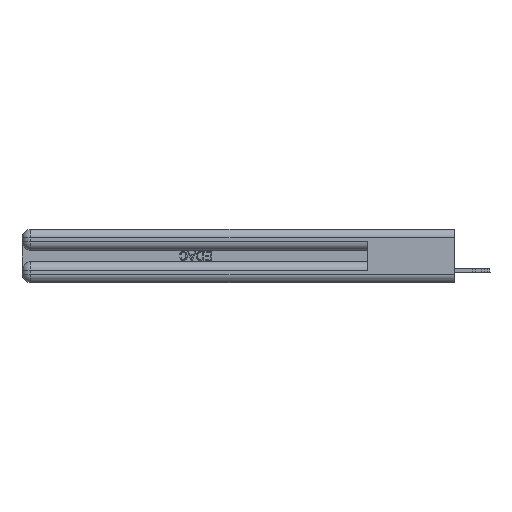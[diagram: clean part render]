
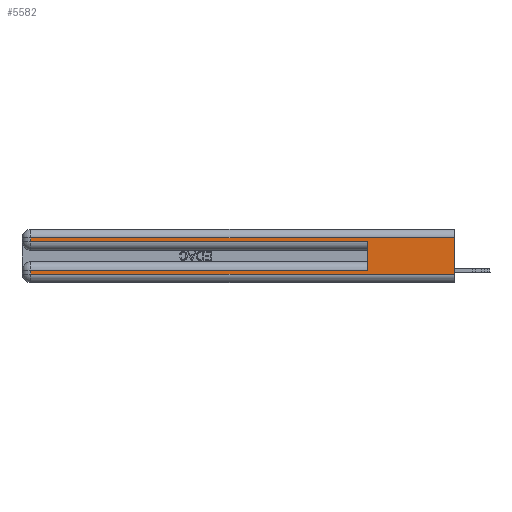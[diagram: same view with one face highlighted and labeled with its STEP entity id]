
A CAD part, left-side view. The second image highlights one B-rep face of the part: STEP entity #5582.
In plain terms, the highlighted planar face has unit normal (-1, 0, 0).
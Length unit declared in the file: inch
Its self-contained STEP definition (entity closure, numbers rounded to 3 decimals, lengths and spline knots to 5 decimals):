
#443 = VECTOR ( 'NONE', #26370, 39.37008 ) ;
#1154 = LINE ( 'NONE', #27697, #9034 ) ;
#2442 = DIRECTION ( 'NONE',  ( 1., 0., 0. ) ) ;
#3306 = VERTEX_POINT ( 'NONE', #29395 ) ;
#4145 = VECTOR ( 'NONE', #40556, 39.37008 ) ;
#4469 = ORIENTED_EDGE ( 'NONE', *, *, #9109, .T. ) ;
#4774 = EDGE_LOOP ( 'NONE', ( #36226, #4469, #39817, #7305, #7699, #21751, #13454, #14660 ) ) ;
#5394 = DIRECTION ( 'NONE',  ( 0., 0., 1. ) ) ;
#5557 = VERTEX_POINT ( 'NONE', #19519 ) ;
#5582 = ADVANCED_FACE ( 'NONE', ( #32559 ), #15690, .F. ) ;
#7305 = ORIENTED_EDGE ( 'NONE', *, *, #16954, .T. ) ;
#7699 = ORIENTED_EDGE ( 'NONE', *, *, #25965, .F. ) ;
#9034 = VECTOR ( 'NONE', #38230, 39.37008 ) ;
#9109 = EDGE_CURVE ( 'NONE', #16203, #12851, #16235, .T. ) ;
#11168 = VECTOR ( 'NONE', #5394, 39.37008 ) ;
#12367 = CARTESIAN_POINT ( 'NONE',  ( 0., 2.94, 0.06 ) ) ;
#12851 = VERTEX_POINT ( 'NONE', #13276 ) ;
#13276 = CARTESIAN_POINT ( 'NONE',  ( 0., 2.94, 0.31 ) ) ;
#13454 = ORIENTED_EDGE ( 'NONE', *, *, #15266, .T. ) ;
#14408 = VECTOR ( 'NONE', #34751, 39.37008 ) ;
#14660 = ORIENTED_EDGE ( 'NONE', *, *, #39453, .T. ) ;
#15266 = EDGE_CURVE ( 'NONE', #39460, #23710, #37892, .T. ) ;
#15690 = PLANE ( 'NONE',  #36865 ) ;
#16203 = VERTEX_POINT ( 'NONE', #29167 ) ;
#16235 = LINE ( 'NONE', #23032, #443 ) ;
#16908 = CARTESIAN_POINT ( 'NONE',  ( 0., 0.6, 0.285 ) ) ;
#16954 = EDGE_CURVE ( 'NONE', #17671, #34526, #23064, .T. ) ;
#17656 = CARTESIAN_POINT ( 'NONE',  ( 0., 0., 0.37 ) ) ;
#17671 = VERTEX_POINT ( 'NONE', #28675 ) ;
#17697 = DIRECTION ( 'NONE',  ( 0., 0., -1. ) ) ;
#19519 = CARTESIAN_POINT ( 'NONE',  ( 0., 0., 0.06 ) ) ;
#19958 = VECTOR ( 'NONE', #39083, 39.37008 ) ;
#20696 = LINE ( 'NONE', #17656, #14408 ) ;
#20820 = EDGE_CURVE ( 'NONE', #12851, #17671, #36679, .T. ) ;
#20942 = CARTESIAN_POINT ( 'NONE',  ( 0., 2.94, 0.37 ) ) ;
#21751 = ORIENTED_EDGE ( 'NONE', *, *, #33394, .T. ) ;
#22437 = CARTESIAN_POINT ( 'NONE',  ( 0., 0., 0.37 ) ) ;
#23032 = CARTESIAN_POINT ( 'NONE',  ( 0., 0., 0.31 ) ) ;
#23064 = LINE ( 'NONE', #39695, #4145 ) ;
#23710 = VERTEX_POINT ( 'NONE', #12367 ) ;
#25199 = EDGE_CURVE ( 'NONE', #16203, #5557, #20696, .T. ) ;
#25965 = EDGE_CURVE ( 'NONE', #3306, #34526, #36319, .T. ) ;
#26370 = DIRECTION ( 'NONE',  ( 0., 1., 0. ) ) ;
#27422 = LINE ( 'NONE', #32650, #33184 ) ;
#27697 = CARTESIAN_POINT ( 'NONE',  ( 0., 0., 0.085 ) ) ;
#28566 = CARTESIAN_POINT ( 'NONE',  ( 0., 0.6, 0.145 ) ) ;
#28675 = CARTESIAN_POINT ( 'NONE',  ( 0., 2.94, 0.285 ) ) ;
#29122 = DIRECTION ( 'NONE',  ( 0., -1., 0. ) ) ;
#29167 = CARTESIAN_POINT ( 'NONE',  ( 0., 0., 0.31 ) ) ;
#29395 = CARTESIAN_POINT ( 'NONE',  ( 0., 0.6, 0.085 ) ) ;
#31629 = VECTOR ( 'NONE', #17697, 39.37008 ) ;
#32559 = FACE_OUTER_BOUND ( 'NONE', #4774, .T. ) ;
#32650 = CARTESIAN_POINT ( 'NONE',  ( 0., 0., 0.06 ) ) ;
#33061 = CARTESIAN_POINT ( 'NONE',  ( 0., 2.94, 0.37 ) ) ;
#33184 = VECTOR ( 'NONE', #29122, 39.37008 ) ;
#33394 = EDGE_CURVE ( 'NONE', #3306, #39460, #1154, .T. ) ;
#34526 = VERTEX_POINT ( 'NONE', #16908 ) ;
#34751 = DIRECTION ( 'NONE',  ( 0., 0., -1. ) ) ;
#35587 = DIRECTION ( 'NONE',  ( 0., 0., -1. ) ) ;
#36226 = ORIENTED_EDGE ( 'NONE', *, *, #25199, .F. ) ;
#36319 = LINE ( 'NONE', #28566, #11168 ) ;
#36679 = LINE ( 'NONE', #33061, #19958 ) ;
#36865 = AXIS2_PLACEMENT_3D ( 'NONE', #22437, #2442, #35587 ) ;
#37892 = LINE ( 'NONE', #20942, #31629 ) ;
#38230 = DIRECTION ( 'NONE',  ( 0., 1., 0. ) ) ;
#39083 = DIRECTION ( 'NONE',  ( 0., 0., -1. ) ) ;
#39453 = EDGE_CURVE ( 'NONE', #23710, #5557, #27422, .T. ) ;
#39460 = VERTEX_POINT ( 'NONE', #42511 ) ;
#39695 = CARTESIAN_POINT ( 'NONE',  ( 0., 0., 0.285 ) ) ;
#39817 = ORIENTED_EDGE ( 'NONE', *, *, #20820, .T. ) ;
#40556 = DIRECTION ( 'NONE',  ( 0., -1., 0. ) ) ;
#42511 = CARTESIAN_POINT ( 'NONE',  ( 0., 2.94, 0.085 ) ) ;
